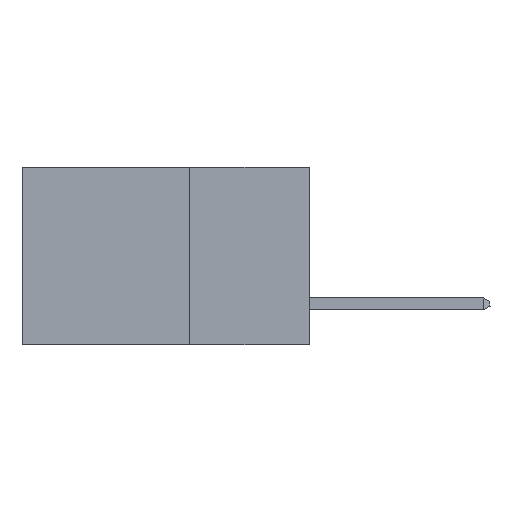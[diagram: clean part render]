
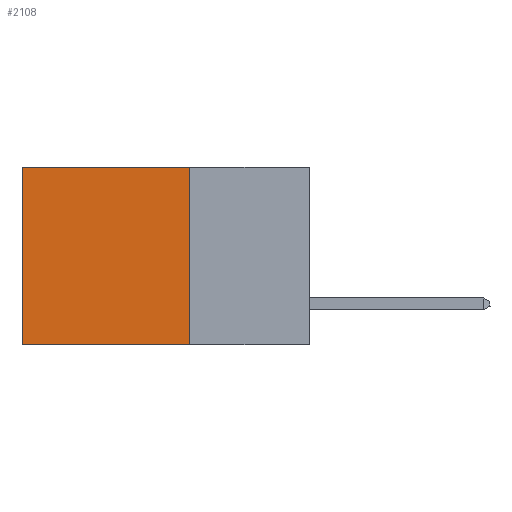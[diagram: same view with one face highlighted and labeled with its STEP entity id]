
A CAD part, left-side view. The second image highlights one B-rep face of the part: STEP entity #2108.
In plain terms, the highlighted planar face has unit normal (-1, 0, 0).
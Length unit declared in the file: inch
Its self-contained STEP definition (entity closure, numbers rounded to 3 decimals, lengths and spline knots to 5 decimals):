
#103 = VECTOR ( 'NONE', #19823, 39.37008 ) ;
#399 = ORIENTED_EDGE ( 'NONE', *, *, #11369, .T. ) ;
#404 = CARTESIAN_POINT ( 'NONE',  ( 0.2875, 0.25, 0. ) ) ;
#1190 = VECTOR ( 'NONE', #9490, 39.37008 ) ;
#1472 = LINE ( 'NONE', #12113, #16569 ) ;
#1651 = VERTEX_POINT ( 'NONE', #21298 ) ;
#1761 = CARTESIAN_POINT ( 'NONE',  ( 0.2875, 0.6, 0. ) ) ;
#2083 = VERTEX_POINT ( 'NONE', #404 ) ;
#2108 = ADVANCED_FACE ( 'NONE', ( #20976 ), #19453, .F. ) ;
#2265 = LINE ( 'NONE', #1761, #1190 ) ;
#3474 = DIRECTION ( 'NONE',  ( 0., 1., 0. ) ) ;
#5940 = VECTOR ( 'NONE', #3474, 39.37008 ) ;
#6472 = VERTEX_POINT ( 'NONE', #11083 ) ;
#6634 = VERTEX_POINT ( 'NONE', #20885 ) ;
#6765 = LINE ( 'NONE', #7074, #5940 ) ;
#7074 = CARTESIAN_POINT ( 'NONE',  ( 0.2875, 0.25, -0.37 ) ) ;
#9490 = DIRECTION ( 'NONE',  ( 0., 0., -1. ) ) ;
#9839 = LINE ( 'NONE', #15419, #103 ) ;
#10711 = CARTESIAN_POINT ( 'NONE',  ( 0.2875, 0.25, 0. ) ) ;
#11083 = CARTESIAN_POINT ( 'NONE',  ( 0.2875, 0.25, -0.37 ) ) ;
#11369 = EDGE_CURVE ( 'NONE', #2083, #6634, #9839, .T. ) ;
#12015 = ORIENTED_EDGE ( 'NONE', *, *, #21733, .F. ) ;
#12113 = CARTESIAN_POINT ( 'NONE',  ( 0.2875, 0.25, 0. ) ) ;
#13316 = AXIS2_PLACEMENT_3D ( 'NONE', #10711, #17439, #17735 ) ;
#13868 = DIRECTION ( 'NONE',  ( 0., 0., -1. ) ) ;
#15419 = CARTESIAN_POINT ( 'NONE',  ( 0.2875, 0.25, 0. ) ) ;
#15928 = EDGE_CURVE ( 'NONE', #6634, #1651, #2265, .T. ) ;
#16569 = VECTOR ( 'NONE', #13868, 39.37008 ) ;
#16734 = EDGE_CURVE ( 'NONE', #6472, #1651, #6765, .T. ) ;
#17439 = DIRECTION ( 'NONE',  ( 1., 0., 0. ) ) ;
#17735 = DIRECTION ( 'NONE',  ( 0., 0., -1. ) ) ;
#19341 = ORIENTED_EDGE ( 'NONE', *, *, #16734, .F. ) ;
#19453 = PLANE ( 'NONE',  #13316 ) ;
#19823 = DIRECTION ( 'NONE',  ( 0., 1., 0. ) ) ;
#20647 = EDGE_LOOP ( 'NONE', ( #21490, #19341, #12015, #399 ) ) ;
#20885 = CARTESIAN_POINT ( 'NONE',  ( 0.2875, 0.6, 0. ) ) ;
#20976 = FACE_OUTER_BOUND ( 'NONE', #20647, .T. ) ;
#21298 = CARTESIAN_POINT ( 'NONE',  ( 0.2875, 0.6, -0.37 ) ) ;
#21490 = ORIENTED_EDGE ( 'NONE', *, *, #15928, .T. ) ;
#21733 = EDGE_CURVE ( 'NONE', #2083, #6472, #1472, .T. ) ;
